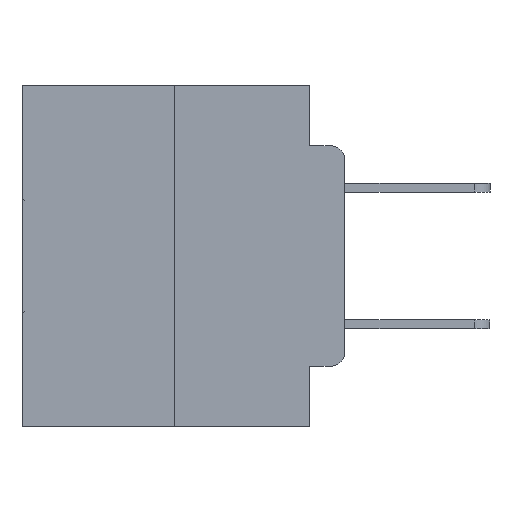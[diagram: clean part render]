
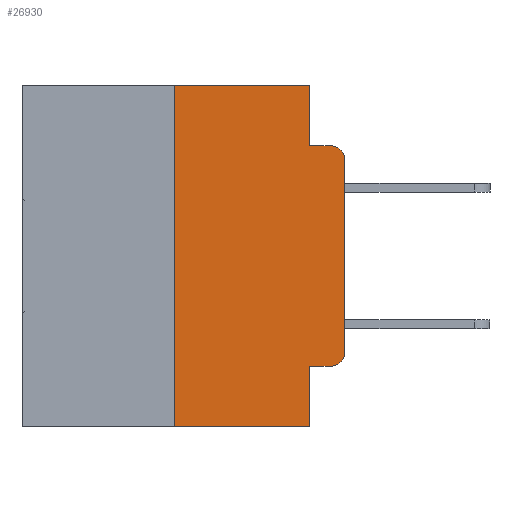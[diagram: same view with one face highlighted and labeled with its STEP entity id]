
A CAD part, left-side view. The second image highlights one B-rep face of the part: STEP entity #26930.
In plain terms, the highlighted planar face has unit normal (-1, 0, 0).
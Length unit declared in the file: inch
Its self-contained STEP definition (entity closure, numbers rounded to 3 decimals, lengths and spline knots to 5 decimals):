
#21 = VECTOR ( 'NONE', #19997, 39.37008 ) ;
#46 = ORIENTED_EDGE ( 'NONE', *, *, #11334, .T. ) ;
#430 = LINE ( 'NONE', #19070, #23574 ) ;
#858 = ORIENTED_EDGE ( 'NONE', *, *, #23592, .T. ) ;
#1126 = FACE_OUTER_BOUND ( 'NONE', #20831, .T. ) ;
#1348 = DIRECTION ( 'NONE',  ( 0., 0., -1. ) ) ;
#1392 = VECTOR ( 'NONE', #13924, 39.37008 ) ;
#1514 = LINE ( 'NONE', #6229, #21 ) ;
#1821 = CARTESIAN_POINT ( 'NONE',  ( 0., 0.473, 0. ) ) ;
#1828 = VERTEX_POINT ( 'NONE', #24265 ) ;
#3232 = VECTOR ( 'NONE', #21401, 39.37008 ) ;
#3456 = VERTEX_POINT ( 'NONE', #25170 ) ;
#3501 = VERTEX_POINT ( 'NONE', #27501 ) ;
#3820 = ORIENTED_EDGE ( 'NONE', *, *, #26603, .T. ) ;
#4123 = CARTESIAN_POINT ( 'NONE',  ( 0., 0.473, 0. ) ) ;
#4347 = AXIS2_PLACEMENT_3D ( 'NONE', #22954, #9243, #25207 ) ;
#4602 = LINE ( 'NONE', #19121, #17513 ) ;
#5350 = DIRECTION ( 'NONE',  ( 0., 0., 1. ) ) ;
#5610 = VERTEX_POINT ( 'NONE', #26941 ) ;
#6229 = CARTESIAN_POINT ( 'NONE',  ( 0., 0.25, 0. ) ) ;
#6618 = ORIENTED_EDGE ( 'NONE', *, *, #24453, .T. ) ;
#6623 = LINE ( 'NONE', #8545, #18141 ) ;
#7919 = ORIENTED_EDGE ( 'NONE', *, *, #17515, .F. ) ;
#8545 = CARTESIAN_POINT ( 'NONE',  ( 0., 0.051, 0. ) ) ;
#8912 = CARTESIAN_POINT ( 'NONE',  ( 0., 0.25, -0.5 ) ) ;
#9124 = VECTOR ( 'NONE', #18929, 39.37008 ) ;
#9243 = DIRECTION ( 'NONE',  ( -1., 0., 0. ) ) ;
#9425 = VERTEX_POINT ( 'NONE', #18159 ) ;
#9580 = AXIS2_PLACEMENT_3D ( 'NONE', #28766, #15327, #1348 ) ;
#11027 = DIRECTION ( 'NONE',  ( 1., 0., 0. ) ) ;
#11098 = DIRECTION ( 'NONE',  ( 0., -1., 0. ) ) ;
#11334 = EDGE_CURVE ( 'NONE', #15512, #9425, #17017, .T. ) ;
#11378 = ORIENTED_EDGE ( 'NONE', *, *, #27570, .F. ) ;
#12066 = CARTESIAN_POINT ( 'NONE',  ( 0., 0.051, -0.0885 ) ) ;
#12295 = CARTESIAN_POINT ( 'NONE',  ( 0., 0.051, 0. ) ) ;
#12740 = ORIENTED_EDGE ( 'NONE', *, *, #12886, .T. ) ;
#12886 = EDGE_CURVE ( 'NONE', #3456, #15512, #20609, .T. ) ;
#13261 = PLANE ( 'NONE',  #19596 ) ;
#13924 = DIRECTION ( 'NONE',  ( 0., -1., 0. ) ) ;
#14287 = VECTOR ( 'NONE', #11098, 39.37008 ) ;
#14492 = EDGE_CURVE ( 'NONE', #3456, #5610, #14838, .T. ) ;
#14838 = LINE ( 'NONE', #12295, #3232 ) ;
#15276 = LINE ( 'NONE', #12066, #9124 ) ;
#15327 = DIRECTION ( 'NONE',  ( -1., 0., 0. ) ) ;
#15512 = VERTEX_POINT ( 'NONE', #27517 ) ;
#16100 = ORIENTED_EDGE ( 'NONE', *, *, #14492, .F. ) ;
#16137 = VERTEX_POINT ( 'NONE', #23900 ) ;
#16187 = CIRCLE ( 'NONE', #4347, 0.02 ) ;
#17017 = CIRCLE ( 'NONE', #9580, 0.02 ) ;
#17513 = VECTOR ( 'NONE', #5350, 39.37008 ) ;
#17515 = EDGE_CURVE ( 'NONE', #27590, #16137, #1514, .T. ) ;
#18141 = VECTOR ( 'NONE', #24518, 39.37008 ) ;
#18159 = CARTESIAN_POINT ( 'NONE',  ( 0., 0., -0.3915 ) ) ;
#18929 = DIRECTION ( 'NONE',  ( 0., -1., 0. ) ) ;
#19055 = ORIENTED_EDGE ( 'NONE', *, *, #19075, .F. ) ;
#19070 = CARTESIAN_POINT ( 'NONE',  ( 0., 0.473, -0.5 ) ) ;
#19075 = EDGE_CURVE ( 'NONE', #24845, #1828, #6623, .T. ) ;
#19121 = CARTESIAN_POINT ( 'NONE',  ( 0., 0., 0. ) ) ;
#19596 = AXIS2_PLACEMENT_3D ( 'NONE', #4123, #11027, #26954 ) ;
#19997 = DIRECTION ( 'NONE',  ( 0., 0., 1. ) ) ;
#20591 = EDGE_CURVE ( 'NONE', #1828, #3501, #15276, .T. ) ;
#20609 = LINE ( 'NONE', #27466, #1392 ) ;
#20662 = CARTESIAN_POINT ( 'NONE',  ( 0., 0., -0.1085 ) ) ;
#20831 = EDGE_LOOP ( 'NONE', ( #3820, #858, #28049, #19055, #11378, #7919, #6618, #16100, #12740, #46 ) ) ;
#21401 = DIRECTION ( 'NONE',  ( 0., 0., -1. ) ) ;
#22337 = VERTEX_POINT ( 'NONE', #20662 ) ;
#22954 = CARTESIAN_POINT ( 'NONE',  ( 0., 0.02, -0.1085 ) ) ;
#23574 = VECTOR ( 'NONE', #23590, 39.37008 ) ;
#23590 = DIRECTION ( 'NONE',  ( 0., -1., 0. ) ) ;
#23592 = EDGE_CURVE ( 'NONE', #22337, #3501, #16187, .T. ) ;
#23900 = CARTESIAN_POINT ( 'NONE',  ( 0., 0.25, 0. ) ) ;
#24265 = CARTESIAN_POINT ( 'NONE',  ( 0., 0.051, -0.0885 ) ) ;
#24453 = EDGE_CURVE ( 'NONE', #27590, #5610, #430, .T. ) ;
#24518 = DIRECTION ( 'NONE',  ( 0., 0., -1. ) ) ;
#24845 = VERTEX_POINT ( 'NONE', #28011 ) ;
#25170 = CARTESIAN_POINT ( 'NONE',  ( 0., 0.051, -0.4115 ) ) ;
#25207 = DIRECTION ( 'NONE',  ( 0., 0., -1. ) ) ;
#26314 = LINE ( 'NONE', #1821, #14287 ) ;
#26603 = EDGE_CURVE ( 'NONE', #9425, #22337, #4602, .T. ) ;
#26930 = ADVANCED_FACE ( 'NONE', ( #1126 ), #13261, .F. ) ;
#26941 = CARTESIAN_POINT ( 'NONE',  ( 0., 0.051, -0.5 ) ) ;
#26954 = DIRECTION ( 'NONE',  ( 0., 0., -1. ) ) ;
#27466 = CARTESIAN_POINT ( 'NONE',  ( 0., 0.051, -0.4115 ) ) ;
#27501 = CARTESIAN_POINT ( 'NONE',  ( 0., 0.02, -0.0885 ) ) ;
#27517 = CARTESIAN_POINT ( 'NONE',  ( 0., 0.02, -0.4115 ) ) ;
#27570 = EDGE_CURVE ( 'NONE', #16137, #24845, #26314, .T. ) ;
#27590 = VERTEX_POINT ( 'NONE', #8912 ) ;
#28011 = CARTESIAN_POINT ( 'NONE',  ( 0., 0.051, 0. ) ) ;
#28049 = ORIENTED_EDGE ( 'NONE', *, *, #20591, .F. ) ;
#28766 = CARTESIAN_POINT ( 'NONE',  ( 0., 0.02, -0.3915 ) ) ;
